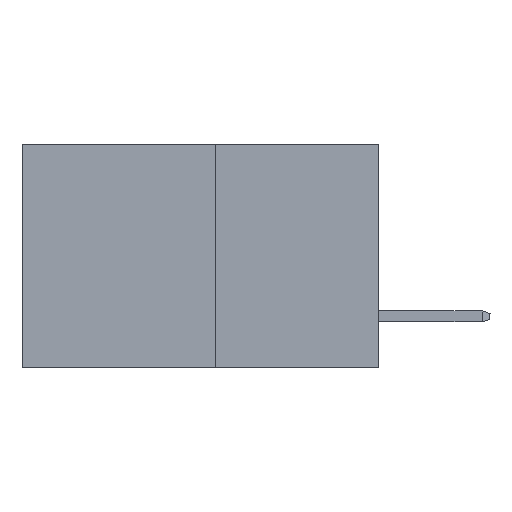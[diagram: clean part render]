
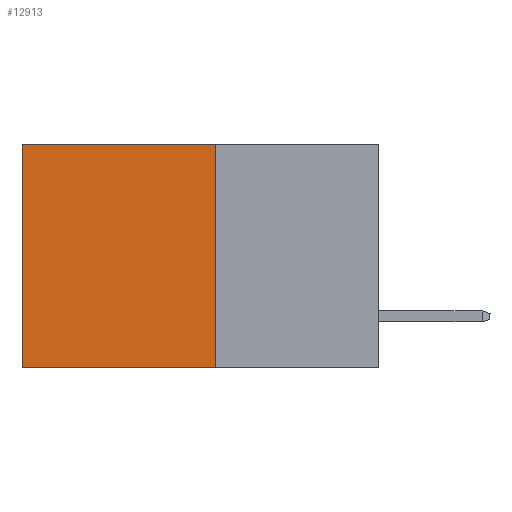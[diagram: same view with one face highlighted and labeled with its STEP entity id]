
A CAD part, left-side view. The second image highlights one B-rep face of the part: STEP entity #12913.
In plain terms, the highlighted planar face has unit normal (-1, 0, 0).
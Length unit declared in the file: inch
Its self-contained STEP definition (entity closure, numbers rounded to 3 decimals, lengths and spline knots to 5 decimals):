
#322 = DIRECTION ( 'NONE',  ( 1., 0., 0. ) ) ;
#1294 = CARTESIAN_POINT ( 'NONE',  ( 0.277, 0.27, 0. ) ) ;
#1419 = LINE ( 'NONE', #9119, #6766 ) ;
#1535 = CARTESIAN_POINT ( 'NONE',  ( 0.277, 0.27, -0.37 ) ) ;
#2213 = LINE ( 'NONE', #14036, #7896 ) ;
#2347 = VERTEX_POINT ( 'NONE', #13401 ) ;
#2405 = CARTESIAN_POINT ( 'NONE',  ( 0.277, 0.59, -0.37 ) ) ;
#2481 = DIRECTION ( 'NONE',  ( 0., 1., 0. ) ) ;
#3474 = AXIS2_PLACEMENT_3D ( 'NONE', #11529, #322, #8278 ) ;
#5254 = LINE ( 'NONE', #1294, #11199 ) ;
#5583 = ORIENTED_EDGE ( 'NONE', *, *, #10624, .F. ) ;
#5847 = LINE ( 'NONE', #1535, #7450 ) ;
#5939 = ORIENTED_EDGE ( 'NONE', *, *, #11337, .F. ) ;
#6104 = ORIENTED_EDGE ( 'NONE', *, *, #7744, .T. ) ;
#6438 = EDGE_CURVE ( 'NONE', #7168, #2347, #5254, .T. ) ;
#6766 = VECTOR ( 'NONE', #11311, 39.37008 ) ;
#7168 = VERTEX_POINT ( 'NONE', #7733 ) ;
#7175 = PLANE ( 'NONE',  #3474 ) ;
#7450 = VECTOR ( 'NONE', #8319, 39.37008 ) ;
#7733 = CARTESIAN_POINT ( 'NONE',  ( 0.277, 0.27, 0. ) ) ;
#7744 = EDGE_CURVE ( 'NONE', #2347, #9555, #2213, .T. ) ;
#7896 = VECTOR ( 'NONE', #9804, 39.37008 ) ;
#8278 = DIRECTION ( 'NONE',  ( 0., 0., -1. ) ) ;
#8319 = DIRECTION ( 'NONE',  ( 0., 0., -1. ) ) ;
#8676 = FACE_OUTER_BOUND ( 'NONE', #12613, .T. ) ;
#9119 = CARTESIAN_POINT ( 'NONE',  ( 0.277, 0.27, -0.37 ) ) ;
#9555 = VERTEX_POINT ( 'NONE', #2405 ) ;
#9804 = DIRECTION ( 'NONE',  ( 0., 0., -1. ) ) ;
#10624 = EDGE_CURVE ( 'NONE', #14396, #9555, #1419, .T. ) ;
#11199 = VECTOR ( 'NONE', #2481, 39.37008 ) ;
#11311 = DIRECTION ( 'NONE',  ( 0., 1., 0. ) ) ;
#11337 = EDGE_CURVE ( 'NONE', #7168, #14396, #5847, .T. ) ;
#11529 = CARTESIAN_POINT ( 'NONE',  ( 0.277, 0.27, -0.37 ) ) ;
#12134 = ORIENTED_EDGE ( 'NONE', *, *, #6438, .T. ) ;
#12613 = EDGE_LOOP ( 'NONE', ( #6104, #5583, #5939, #12134 ) ) ;
#12637 = CARTESIAN_POINT ( 'NONE',  ( 0.277, 0.27, -0.37 ) ) ;
#12913 = ADVANCED_FACE ( 'NONE', ( #8676 ), #7175, .F. ) ;
#13401 = CARTESIAN_POINT ( 'NONE',  ( 0.277, 0.59, 0. ) ) ;
#14036 = CARTESIAN_POINT ( 'NONE',  ( 0.277, 0.59, -0.37 ) ) ;
#14396 = VERTEX_POINT ( 'NONE', #12637 ) ;
